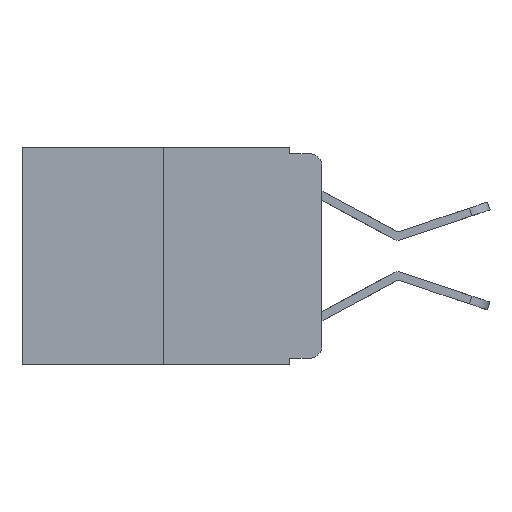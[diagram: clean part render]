
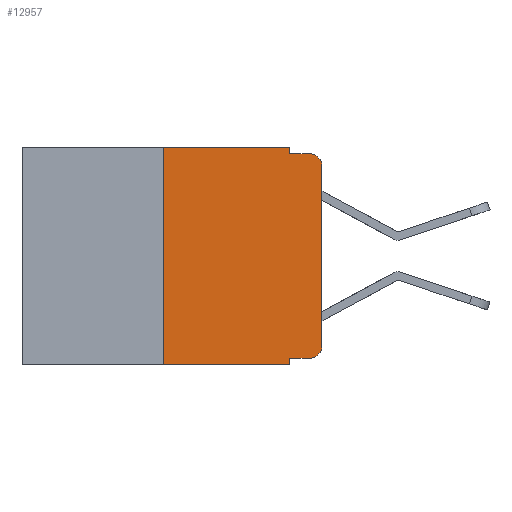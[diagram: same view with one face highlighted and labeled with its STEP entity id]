
A CAD part, left-side view. The second image highlights one B-rep face of the part: STEP entity #12957.
In plain terms, the highlighted planar face has unit normal (-1, 0, 0).
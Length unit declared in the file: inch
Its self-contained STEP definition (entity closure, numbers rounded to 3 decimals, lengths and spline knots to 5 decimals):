
#359 = CARTESIAN_POINT ( 'NONE',  ( 0., 0.051, -0.01 ) ) ;
#416 = CARTESIAN_POINT ( 'NONE',  ( 0., 0.051, -0.01 ) ) ;
#541 = DIRECTION ( 'NONE',  ( 0., 0., -1. ) ) ;
#585 = CARTESIAN_POINT ( 'NONE',  ( 0., 0., -0.313 ) ) ;
#656 = DIRECTION ( 'NONE',  ( -1., 0., 0. ) ) ;
#930 = DIRECTION ( 'NONE',  ( 0., 0., -1. ) ) ;
#1024 = VERTEX_POINT ( 'NONE', #9017 ) ;
#1238 = DIRECTION ( 'NONE',  ( 0., -1., 0. ) ) ;
#1377 = EDGE_CURVE ( 'NONE', #11182, #10442, #12777, .T. ) ;
#1389 = EDGE_CURVE ( 'NONE', #1024, #1675, #2251, .T. ) ;
#1514 = EDGE_CURVE ( 'NONE', #10442, #12180, #12447, .T. ) ;
#1530 = DIRECTION ( 'NONE',  ( 0., -1., 0. ) ) ;
#1675 = VERTEX_POINT ( 'NONE', #359 ) ;
#1722 = ORIENTED_EDGE ( 'NONE', *, *, #2944, .F. ) ;
#1808 = DIRECTION ( 'NONE',  ( 0., 0., -1. ) ) ;
#1967 = DIRECTION ( 'NONE',  ( 0., 0., -1. ) ) ;
#2036 = FACE_OUTER_BOUND ( 'NONE', #13046, .T. ) ;
#2149 = DIRECTION ( 'NONE',  ( 0., -1., 0. ) ) ;
#2229 = LINE ( 'NONE', #416, #7442 ) ;
#2251 = LINE ( 'NONE', #9002, #4763 ) ;
#2362 = VERTEX_POINT ( 'NONE', #10857 ) ;
#2480 = VERTEX_POINT ( 'NONE', #9413 ) ;
#2594 = ORIENTED_EDGE ( 'NONE', *, *, #10582, .T. ) ;
#2944 = EDGE_CURVE ( 'NONE', #4146, #2480, #5340, .T. ) ;
#3093 = DIRECTION ( 'NONE',  ( -1., 0., 0. ) ) ;
#3107 = LINE ( 'NONE', #4136, #11219 ) ;
#3233 = CARTESIAN_POINT ( 'NONE',  ( 0., 0.02, -0.333 ) ) ;
#3405 = VERTEX_POINT ( 'NONE', #3233 ) ;
#3616 = AXIS2_PLACEMENT_3D ( 'NONE', #7018, #656, #8012 ) ;
#4088 = ORIENTED_EDGE ( 'NONE', *, *, #5142, .T. ) ;
#4136 = CARTESIAN_POINT ( 'NONE',  ( 0., 0.051, 0. ) ) ;
#4146 = VERTEX_POINT ( 'NONE', #6722 ) ;
#4664 = EDGE_CURVE ( 'NONE', #4146, #10261, #8584, .T. ) ;
#4744 = DIRECTION ( 'NONE',  ( 0., 0., 1. ) ) ;
#4763 = VECTOR ( 'NONE', #541, 39.37008 ) ;
#4995 = CIRCLE ( 'NONE', #3616, 0.02 ) ;
#5142 = EDGE_CURVE ( 'NONE', #2362, #3405, #6546, .T. ) ;
#5340 = LINE ( 'NONE', #9515, #10666 ) ;
#5876 = ORIENTED_EDGE ( 'NONE', *, *, #4664, .T. ) ;
#5922 = VECTOR ( 'NONE', #10721, 39.37008 ) ;
#6015 = PLANE ( 'NONE',  #11779 ) ;
#6023 = ORIENTED_EDGE ( 'NONE', *, *, #6237, .F. ) ;
#6237 = EDGE_CURVE ( 'NONE', #2480, #1024, #9840, .T. ) ;
#6314 = ORIENTED_EDGE ( 'NONE', *, *, #1514, .T. ) ;
#6546 = LINE ( 'NONE', #7533, #13261 ) ;
#6666 = CARTESIAN_POINT ( 'NONE',  ( 0., 0.02, -0.01 ) ) ;
#6722 = CARTESIAN_POINT ( 'NONE',  ( 0., 0.25, -0.343 ) ) ;
#7018 = CARTESIAN_POINT ( 'NONE',  ( 0., 0.02, -0.313 ) ) ;
#7055 = CARTESIAN_POINT ( 'NONE',  ( 0., 0.473, 0. ) ) ;
#7196 = VECTOR ( 'NONE', #2149, 39.37008 ) ;
#7276 = ORIENTED_EDGE ( 'NONE', *, *, #12271, .F. ) ;
#7442 = VECTOR ( 'NONE', #1530, 39.37008 ) ;
#7533 = CARTESIAN_POINT ( 'NONE',  ( 0., 0.051, -0.333 ) ) ;
#7603 = EDGE_CURVE ( 'NONE', #2362, #10261, #3107, .T. ) ;
#8012 = DIRECTION ( 'NONE',  ( 0., 0., -1. ) ) ;
#8045 = DIRECTION ( 'NONE',  ( 1., 0., 0. ) ) ;
#8349 = CARTESIAN_POINT ( 'NONE',  ( 0., 0.473, 0. ) ) ;
#8584 = LINE ( 'NONE', #8722, #5922 ) ;
#8722 = CARTESIAN_POINT ( 'NONE',  ( 0., 0.473, -0.343 ) ) ;
#9002 = CARTESIAN_POINT ( 'NONE',  ( 0., 0.051, 0. ) ) ;
#9017 = CARTESIAN_POINT ( 'NONE',  ( 0., 0.051, 0. ) ) ;
#9412 = CARTESIAN_POINT ( 'NONE',  ( 0., 0.051, -0.343 ) ) ;
#9413 = CARTESIAN_POINT ( 'NONE',  ( 0., 0.25, 0. ) ) ;
#9515 = CARTESIAN_POINT ( 'NONE',  ( 0., 0.25, 0. ) ) ;
#9630 = CARTESIAN_POINT ( 'NONE',  ( 0., 0., 0. ) ) ;
#9840 = LINE ( 'NONE', #8349, #7196 ) ;
#10261 = VERTEX_POINT ( 'NONE', #9412 ) ;
#10442 = VERTEX_POINT ( 'NONE', #10753 ) ;
#10582 = EDGE_CURVE ( 'NONE', #3405, #11182, #4995, .T. ) ;
#10666 = VECTOR ( 'NONE', #4744, 39.37008 ) ;
#10721 = DIRECTION ( 'NONE',  ( 0., -1., 0. ) ) ;
#10753 = CARTESIAN_POINT ( 'NONE',  ( 0., 0., -0.03 ) ) ;
#10857 = CARTESIAN_POINT ( 'NONE',  ( 0., 0.051, -0.333 ) ) ;
#10861 = CARTESIAN_POINT ( 'NONE',  ( 0., 0.02, -0.03 ) ) ;
#10960 = AXIS2_PLACEMENT_3D ( 'NONE', #10861, #3093, #930 ) ;
#11182 = VERTEX_POINT ( 'NONE', #585 ) ;
#11219 = VECTOR ( 'NONE', #1967, 39.37008 ) ;
#11333 = ORIENTED_EDGE ( 'NONE', *, *, #1377, .T. ) ;
#11779 = AXIS2_PLACEMENT_3D ( 'NONE', #7055, #8045, #1808 ) ;
#11825 = DIRECTION ( 'NONE',  ( 0., 0., 1. ) ) ;
#11830 = ORIENTED_EDGE ( 'NONE', *, *, #7603, .F. ) ;
#12124 = ORIENTED_EDGE ( 'NONE', *, *, #1389, .F. ) ;
#12180 = VERTEX_POINT ( 'NONE', #6666 ) ;
#12271 = EDGE_CURVE ( 'NONE', #1675, #12180, #2229, .T. ) ;
#12447 = CIRCLE ( 'NONE', #10960, 0.02 ) ;
#12677 = VECTOR ( 'NONE', #11825, 39.37008 ) ;
#12777 = LINE ( 'NONE', #9630, #12677 ) ;
#12957 = ADVANCED_FACE ( 'NONE', ( #2036 ), #6015, .F. ) ;
#13046 = EDGE_LOOP ( 'NONE', ( #11333, #6314, #7276, #12124, #6023, #1722, #5876, #11830, #4088, #2594 ) ) ;
#13261 = VECTOR ( 'NONE', #1238, 39.37008 ) ;
